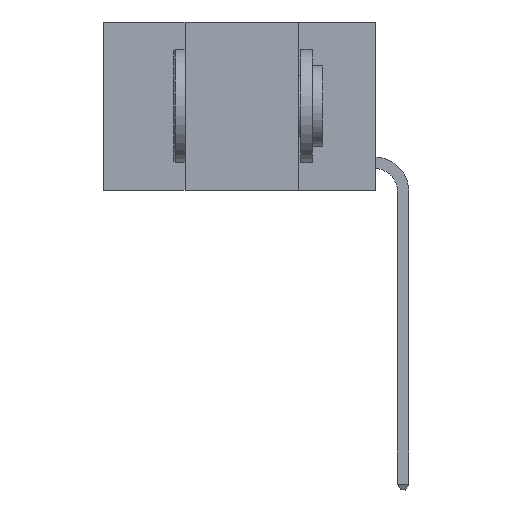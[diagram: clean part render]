
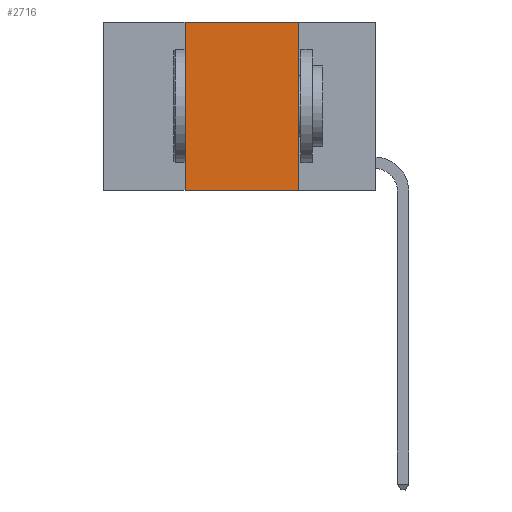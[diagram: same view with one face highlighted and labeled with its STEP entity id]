
A CAD part, left-side view. The second image highlights one B-rep face of the part: STEP entity #2716.
In plain terms, the highlighted planar face has unit normal (-1, 0, 0).
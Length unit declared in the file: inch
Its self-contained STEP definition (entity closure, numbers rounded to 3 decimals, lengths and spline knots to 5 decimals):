
#506 = CARTESIAN_POINT ( 'NONE',  ( 0., 0.17, 0. ) ) ;
#1536 = DIRECTION ( 'NONE',  ( 0., 0., -1. ) ) ;
#2297 = EDGE_CURVE ( 'NONE', #13592, #6755, #5489, .T. ) ;
#2312 = CARTESIAN_POINT ( 'NONE',  ( 0., 0.42, -0.37 ) ) ;
#2328 = AXIS2_PLACEMENT_3D ( 'NONE', #10017, #11734, #1536 ) ;
#2716 = ADVANCED_FACE ( 'NONE', ( #12906 ), #20222, .F. ) ;
#3575 = VERTEX_POINT ( 'NONE', #2312 ) ;
#3941 = DIRECTION ( 'NONE',  ( 0., 0., -1. ) ) ;
#4388 = CARTESIAN_POINT ( 'NONE',  ( 0., 0.42, 0. ) ) ;
#4456 = DIRECTION ( 'NONE',  ( 0., -1., 0. ) ) ;
#5481 = EDGE_LOOP ( 'NONE', ( #6443, #8721, #21195, #21764 ) ) ;
#5489 = LINE ( 'NONE', #506, #11879 ) ;
#5606 = LINE ( 'NONE', #7694, #14643 ) ;
#6005 = CARTESIAN_POINT ( 'NONE',  ( 0., 0.17, 0. ) ) ;
#6096 = CARTESIAN_POINT ( 'NONE',  ( 0., 0.6, 0. ) ) ;
#6443 = ORIENTED_EDGE ( 'NONE', *, *, #2297, .F. ) ;
#6740 = VECTOR ( 'NONE', #7689, 39.37008 ) ;
#6755 = VERTEX_POINT ( 'NONE', #14691 ) ;
#7689 = DIRECTION ( 'NONE',  ( 0., -1., 0. ) ) ;
#7694 = CARTESIAN_POINT ( 'NONE',  ( 0., 0.42, 0. ) ) ;
#8721 = ORIENTED_EDGE ( 'NONE', *, *, #15024, .F. ) ;
#9540 = VECTOR ( 'NONE', #4456, 39.37008 ) ;
#10017 = CARTESIAN_POINT ( 'NONE',  ( 0., 0.6, 0. ) ) ;
#11734 = DIRECTION ( 'NONE',  ( 1., 0., 0. ) ) ;
#11879 = VECTOR ( 'NONE', #3941, 39.37008 ) ;
#12187 = EDGE_CURVE ( 'NONE', #3575, #6755, #19039, .T. ) ;
#12906 = FACE_OUTER_BOUND ( 'NONE', #5481, .T. ) ;
#13021 = VERTEX_POINT ( 'NONE', #4388 ) ;
#13592 = VERTEX_POINT ( 'NONE', #6005 ) ;
#14063 = LINE ( 'NONE', #6096, #9540 ) ;
#14643 = VECTOR ( 'NONE', #21264, 39.37008 ) ;
#14691 = CARTESIAN_POINT ( 'NONE',  ( 0., 0.17, -0.37 ) ) ;
#15024 = EDGE_CURVE ( 'NONE', #13021, #13592, #14063, .T. ) ;
#17894 = CARTESIAN_POINT ( 'NONE',  ( 0., 0.6, -0.37 ) ) ;
#19039 = LINE ( 'NONE', #17894, #6740 ) ;
#20010 = EDGE_CURVE ( 'NONE', #3575, #13021, #5606, .T. ) ;
#20222 = PLANE ( 'NONE',  #2328 ) ;
#21195 = ORIENTED_EDGE ( 'NONE', *, *, #20010, .F. ) ;
#21264 = DIRECTION ( 'NONE',  ( 0., 0., 1. ) ) ;
#21764 = ORIENTED_EDGE ( 'NONE', *, *, #12187, .T. ) ;
